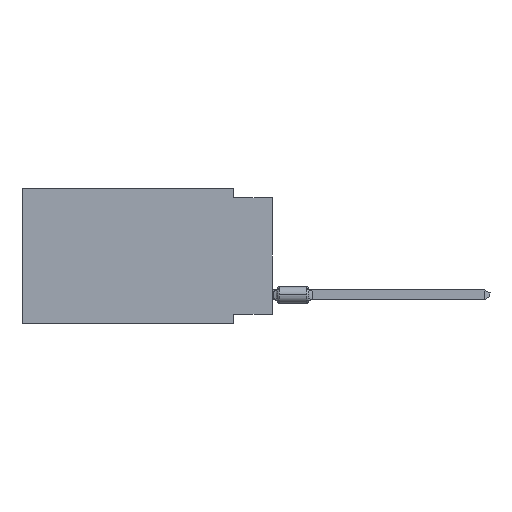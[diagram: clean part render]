
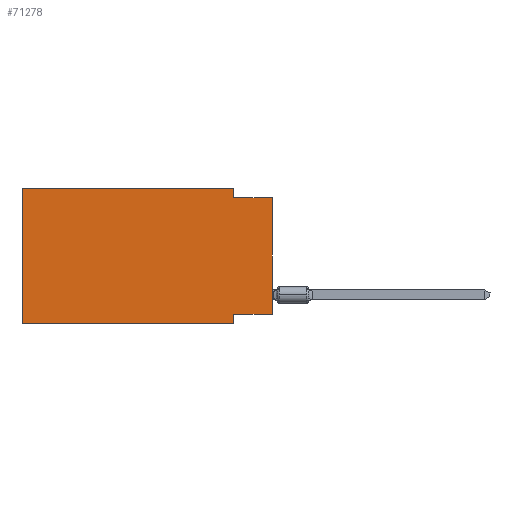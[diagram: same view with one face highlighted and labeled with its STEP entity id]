
A CAD part, left-side view. The second image highlights one B-rep face of the part: STEP entity #71278.
In plain terms, the highlighted planar face has unit normal (-1, 0, 0).
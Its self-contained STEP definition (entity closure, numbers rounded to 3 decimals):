
#2625 = CARTESIAN_POINT ( 'NONE',  ( 0., 16.383, -8.89 ) ) ;
#3951 = VERTEX_POINT ( 'NONE', #73258 ) ;
#6413 = CARTESIAN_POINT ( 'NONE',  ( 0., 0., 0. ) ) ;
#9985 = VERTEX_POINT ( 'NONE', #43644 ) ;
#10332 = VERTEX_POINT ( 'NONE', #71965 ) ;
#14112 = VECTOR ( 'NONE', #45690, 1000. ) ;
#14928 = DIRECTION ( 'NONE',  ( 0., 1., 0. ) ) ;
#16285 = VECTOR ( 'NONE', #84714, 1000. ) ;
#18840 = VERTEX_POINT ( 'NONE', #46783 ) ;
#19459 = DIRECTION ( 'NONE',  ( 0., 0., -1. ) ) ;
#20081 = EDGE_CURVE ( 'NONE', #9985, #18840, #31721, .T. ) ;
#21798 = CARTESIAN_POINT ( 'NONE',  ( 0., 2.54, 0. ) ) ;
#24410 = VERTEX_POINT ( 'NONE', #40265 ) ;
#24751 = LINE ( 'NONE', #69963, #51115 ) ;
#28288 = CARTESIAN_POINT ( 'NONE',  ( 0., 16.383, 0. ) ) ;
#29296 = VECTOR ( 'NONE', #60945, 1000. ) ;
#31721 = LINE ( 'NONE', #63381, #16285 ) ;
#35960 = DIRECTION ( 'NONE',  ( 0., 0., 1. ) ) ;
#36991 = EDGE_CURVE ( 'NONE', #80304, #95868, #68723, .T. ) ;
#37619 = ORIENTED_EDGE ( 'NONE', *, *, #73795, .F. ) ;
#38498 = AXIS2_PLACEMENT_3D ( 'NONE', #28288, #66710, #19459 ) ;
#40265 = CARTESIAN_POINT ( 'NONE',  ( 0., 2.54, -0.635 ) ) ;
#43226 = CARTESIAN_POINT ( 'NONE',  ( 0., 16.383, 0. ) ) ;
#43644 = CARTESIAN_POINT ( 'NONE',  ( 0., 16.383, 0. ) ) ;
#43867 = PLANE ( 'NONE',  #38498 ) ;
#43967 = VECTOR ( 'NONE', #97638, 1000. ) ;
#45690 = DIRECTION ( 'NONE',  ( 0., 0., -1. ) ) ;
#46733 = EDGE_CURVE ( 'NONE', #18840, #24410, #77348, .T. ) ;
#46783 = CARTESIAN_POINT ( 'NONE',  ( 0., 2.54, 0. ) ) ;
#49647 = ORIENTED_EDGE ( 'NONE', *, *, #80328, .T. ) ;
#51115 = VECTOR ( 'NONE', #14928, 1000. ) ;
#52690 = FACE_OUTER_BOUND ( 'NONE', #64464, .T. ) ;
#53328 = DIRECTION ( 'NONE',  ( 0., -1., 0. ) ) ;
#53360 = ORIENTED_EDGE ( 'NONE', *, *, #20081, .F. ) ;
#57552 = CARTESIAN_POINT ( 'NONE',  ( 0., 0., -0.635 ) ) ;
#60374 = CARTESIAN_POINT ( 'NONE',  ( 0., 2.54, -8.255 ) ) ;
#60662 = LINE ( 'NONE', #92327, #83619 ) ;
#60945 = DIRECTION ( 'NONE',  ( 0., 0., 1. ) ) ;
#61625 = CARTESIAN_POINT ( 'NONE',  ( 0., 0., -0.635 ) ) ;
#63381 = CARTESIAN_POINT ( 'NONE',  ( 0., 16.383, 0. ) ) ;
#64464 = EDGE_LOOP ( 'NONE', ( #86706, #96951, #77769, #53360, #90511, #49647, #37619, #90262 ) ) ;
#65968 = LINE ( 'NONE', #2625, #43967 ) ;
#66710 = DIRECTION ( 'NONE',  ( 1., 0., 0. ) ) ;
#68552 = VECTOR ( 'NONE', #53328, 1000. ) ;
#68723 = LINE ( 'NONE', #6413, #29296 ) ;
#69963 = CARTESIAN_POINT ( 'NONE',  ( 0., 0., -8.255 ) ) ;
#71278 = ADVANCED_FACE ( 'NONE', ( #52690 ), #43867, .F. ) ;
#71965 = CARTESIAN_POINT ( 'NONE',  ( 0., 2.54, -8.89 ) ) ;
#72797 = VERTEX_POINT ( 'NONE', #60374 ) ;
#73258 = CARTESIAN_POINT ( 'NONE',  ( 0., 16.383, -8.89 ) ) ;
#73795 = EDGE_CURVE ( 'NONE', #72797, #10332, #60662, .T. ) ;
#77348 = LINE ( 'NONE', #21798, #14112 ) ;
#77769 = ORIENTED_EDGE ( 'NONE', *, *, #46733, .F. ) ;
#80304 = VERTEX_POINT ( 'NONE', #98141 ) ;
#80328 = EDGE_CURVE ( 'NONE', #3951, #10332, #65968, .T. ) ;
#82243 = DIRECTION ( 'NONE',  ( 0., 0., -1. ) ) ;
#83619 = VECTOR ( 'NONE', #82243, 1000. ) ;
#84714 = DIRECTION ( 'NONE',  ( 0., -1., 0. ) ) ;
#86706 = ORIENTED_EDGE ( 'NONE', *, *, #36991, .T. ) ;
#90262 = ORIENTED_EDGE ( 'NONE', *, *, #91698, .F. ) ;
#90511 = ORIENTED_EDGE ( 'NONE', *, *, #96919, .F. ) ;
#90989 = LINE ( 'NONE', #43226, #96670 ) ;
#91698 = EDGE_CURVE ( 'NONE', #80304, #72797, #24751, .T. ) ;
#92327 = CARTESIAN_POINT ( 'NONE',  ( 0., 2.54, -8.89 ) ) ;
#93291 = LINE ( 'NONE', #61625, #68552 ) ;
#95868 = VERTEX_POINT ( 'NONE', #57552 ) ;
#96670 = VECTOR ( 'NONE', #35960, 1000. ) ;
#96919 = EDGE_CURVE ( 'NONE', #3951, #9985, #90989, .T. ) ;
#96951 = ORIENTED_EDGE ( 'NONE', *, *, #97823, .F. ) ;
#97638 = DIRECTION ( 'NONE',  ( 0., -1., 0. ) ) ;
#97823 = EDGE_CURVE ( 'NONE', #24410, #95868, #93291, .T. ) ;
#98141 = CARTESIAN_POINT ( 'NONE',  ( 0., 0., -8.255 ) ) ;
